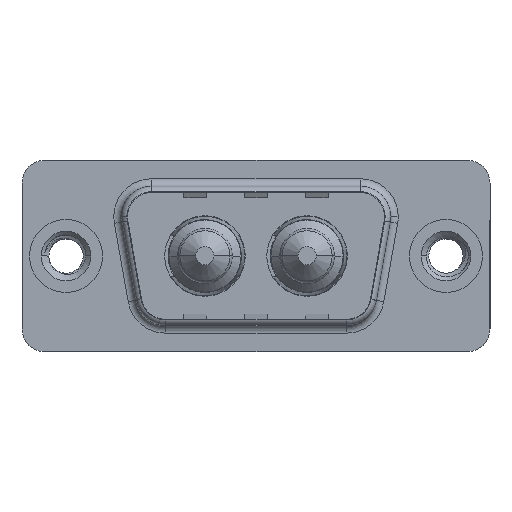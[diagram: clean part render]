
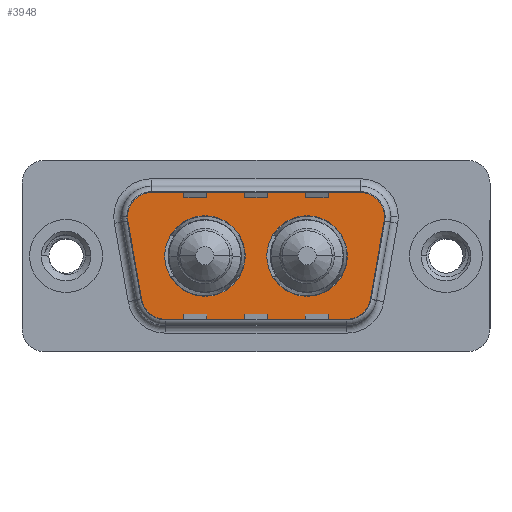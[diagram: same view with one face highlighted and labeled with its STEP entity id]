
A CAD part, top view. The second image highlights one B-rep face of the part: STEP entity #3948.
In plain terms, the highlighted planar face has unit normal (0, 0, 1).
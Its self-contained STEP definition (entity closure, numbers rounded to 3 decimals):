
#132 = CARTESIAN_POINT ( 'NONE',  ( 5.436, 2.9, 0. ) ) ;
#483 = FACE_OUTER_BOUND ( 'NONE', #4924, .T. ) ;
#652 = CARTESIAN_POINT ( 'NONE',  ( 18.51, 0., 0. ) ) ;
#672 = DIRECTION ( 'NONE',  ( 0., 0., 1. ) ) ;
#701 = DIRECTION ( 'NONE',  ( 1., 0., 0. ) ) ;
#782 = VERTEX_POINT ( 'NONE', #12612 ) ;
#841 = EDGE_CURVE ( 'NONE', #10026, #9860, #6600, .T. ) ;
#911 = CARTESIAN_POINT ( 'NONE',  ( 9.14, 0., 0. ) ) ;
#1063 = DIRECTION ( 'NONE',  ( 0., 0., 1. ) ) ;
#1115 = EDGE_CURVE ( 'NONE', #13085, #6826, #3585, .T. ) ;
#1200 = AXIS2_PLACEMENT_3D ( 'NONE', #3878, #1221, #13294 ) ;
#1221 = DIRECTION ( 'NONE',  ( 0., 0., 1. ) ) ;
#1345 = DIRECTION ( 'NONE',  ( 1., 0., 0. ) ) ;
#1602 = ORIENTED_EDGE ( 'NONE', *, *, #3446, .T. ) ;
#1955 = DIRECTION ( 'NONE',  ( 0., 0., 1. ) ) ;
#2204 = CARTESIAN_POINT ( 'NONE',  ( 3.466, 2.553, 0. ) ) ;
#2208 = CARTESIAN_POINT ( 'NONE',  ( 20.511, -3.247, 0. ) ) ;
#2267 = DIRECTION ( 'NONE',  ( -1., 0., 0. ) ) ;
#2275 = PLANE ( 'NONE',  #1200 ) ;
#2322 = ORIENTED_EDGE ( 'NONE', *, *, #5563, .F. ) ;
#2323 = VERTEX_POINT ( 'NONE', #7540 ) ;
#2483 = CARTESIAN_POINT ( 'NONE',  ( 19.564, 2.9, 0. ) ) ;
#2582 = LINE ( 'NONE', #13268, #15132 ) ;
#2843 = CARTESIAN_POINT ( 'NONE',  ( 4.489, -3.247, 0. ) ) ;
#2869 = EDGE_CURVE ( 'NONE', #10676, #13154, #8238, .T. ) ;
#2882 = CIRCLE ( 'NONE', #6363, 2. ) ;
#2895 = CIRCLE ( 'NONE', #12965, 2.65 ) ;
#3183 = CIRCLE ( 'NONE', #9169, 2. ) ;
#3239 = ORIENTED_EDGE ( 'NONE', *, *, #841, .T. ) ;
#3446 = EDGE_CURVE ( 'NONE', #6826, #2323, #2582, .T. ) ;
#3585 = CIRCLE ( 'NONE', #12655, 2. ) ;
#3688 = ORIENTED_EDGE ( 'NONE', *, *, #4561, .T. ) ;
#3711 = FACE_BOUND ( 'NONE', #8739, .T. ) ;
#3712 = DIRECTION ( 'NONE',  ( -1., 0., 0. ) ) ;
#3720 = CARTESIAN_POINT ( 'NONE',  ( 15.86, 0., 0. ) ) ;
#3811 = DIRECTION ( 'NONE',  ( 0., 0., 1. ) ) ;
#3878 = CARTESIAN_POINT ( 'NONE',  ( 18.541, -2.9, 0. ) ) ;
#3948 = ADVANCED_FACE ( 'NONE', ( #13364, #3711, #483 ), #2275, .T. ) ;
#4090 = CARTESIAN_POINT ( 'NONE',  ( 5.436, 4.9, 0. ) ) ;
#4270 = CARTESIAN_POINT ( 'NONE',  ( 11.79, 0., 0. ) ) ;
#4561 = EDGE_CURVE ( 'NONE', #782, #10026, #7264, .T. ) ;
#4793 = CARTESIAN_POINT ( 'NONE',  ( 6.49, 0., 0. ) ) ;
#4800 = CIRCLE ( 'NONE', #15759, 2. ) ;
#4924 = EDGE_LOOP ( 'NONE', ( #15242, #1602, #11312, #3688, #3239, #15595, #5455, #5734, #7598 ) ) ;
#4936 = DIRECTION ( 'NONE',  ( 1., 0., 0. ) ) ;
#5147 = AXIS2_PLACEMENT_3D ( 'NONE', #8876, #11885, #11866 ) ;
#5151 = VERTEX_POINT ( 'NONE', #4793 ) ;
#5455 = ORIENTED_EDGE ( 'NONE', *, *, #2869, .T. ) ;
#5510 = DIRECTION ( 'NONE',  ( 0.174, -0.985, 0. ) ) ;
#5563 = EDGE_CURVE ( 'NONE', #8198, #10175, #7054, .T. ) ;
#5567 = VERTEX_POINT ( 'NONE', #4270 ) ;
#5734 = ORIENTED_EDGE ( 'NONE', *, *, #6696, .T. ) ;
#5757 = EDGE_CURVE ( 'NONE', #2323, #782, #4800, .T. ) ;
#5960 = DIRECTION ( 'NONE',  ( 1., 0., 0. ) ) ;
#5963 = EDGE_CURVE ( 'NONE', #5151, #5567, #2895, .T. ) ;
#6213 = VECTOR ( 'NONE', #2267, 1000. ) ;
#6236 = CARTESIAN_POINT ( 'NONE',  ( 3.466, 2.553, 0. ) ) ;
#6363 = AXIS2_PLACEMENT_3D ( 'NONE', #6787, #6740, #6719 ) ;
#6600 = LINE ( 'NONE', #15587, #6213 ) ;
#6684 = VERTEX_POINT ( 'NONE', #7720 ) ;
#6696 = EDGE_CURVE ( 'NONE', #13154, #6684, #2882, .T. ) ;
#6719 = DIRECTION ( 'NONE',  ( -1., 0., 0. ) ) ;
#6740 = DIRECTION ( 'NONE',  ( 0., 0., 1. ) ) ;
#6787 = CARTESIAN_POINT ( 'NONE',  ( 6.459, -2.9, 0. ) ) ;
#6826 = VERTEX_POINT ( 'NONE', #2208 ) ;
#7026 = CARTESIAN_POINT ( 'NONE',  ( 6.459, -4.9, 0. ) ) ;
#7054 = CIRCLE ( 'NONE', #5147, 2.65 ) ;
#7264 = CIRCLE ( 'NONE', #12854, 2. ) ;
#7540 = CARTESIAN_POINT ( 'NONE',  ( 21.534, 2.553, 0. ) ) ;
#7598 = ORIENTED_EDGE ( 'NONE', *, *, #8894, .T. ) ;
#7692 = VECTOR ( 'NONE', #5960, 1000. ) ;
#7720 = CARTESIAN_POINT ( 'NONE',  ( 6.459, -4.9, 0. ) ) ;
#7918 = EDGE_CURVE ( 'NONE', #9860, #10676, #3183, .T. ) ;
#8198 = VERTEX_POINT ( 'NONE', #652 ) ;
#8238 = LINE ( 'NONE', #6236, #14755 ) ;
#8577 = DIRECTION ( 'NONE',  ( 0., 0., 1. ) ) ;
#8739 = EDGE_LOOP ( 'NONE', ( #12977, #15034 ) ) ;
#8876 = CARTESIAN_POINT ( 'NONE',  ( 15.86, 0., 0. ) ) ;
#8894 = EDGE_CURVE ( 'NONE', #6684, #13085, #15540, .T. ) ;
#9168 = CARTESIAN_POINT ( 'NONE',  ( 9.14, 0., 0. ) ) ;
#9169 = AXIS2_PLACEMENT_3D ( 'NONE', #132, #8577, #1345 ) ;
#9634 = EDGE_LOOP ( 'NONE', ( #2322, #14227 ) ) ;
#9860 = VERTEX_POINT ( 'NONE', #4090 ) ;
#9920 = EDGE_CURVE ( 'NONE', #5567, #5151, #12270, .T. ) ;
#10026 = VERTEX_POINT ( 'NONE', #14216 ) ;
#10175 = VERTEX_POINT ( 'NONE', #10807 ) ;
#10211 = EDGE_CURVE ( 'NONE', #10175, #8198, #12448, .T. ) ;
#10396 = DIRECTION ( 'NONE',  ( 1., 0., 0. ) ) ;
#10676 = VERTEX_POINT ( 'NONE', #2204 ) ;
#10807 = CARTESIAN_POINT ( 'NONE',  ( 13.21, 0., 0. ) ) ;
#11076 = DIRECTION ( 'NONE',  ( 0.174, 0.985, 0. ) ) ;
#11312 = ORIENTED_EDGE ( 'NONE', *, *, #5757, .T. ) ;
#11548 = DIRECTION ( 'NONE',  ( 1., 0., 0. ) ) ;
#11866 = DIRECTION ( 'NONE',  ( 1., 0., 0. ) ) ;
#11885 = DIRECTION ( 'NONE',  ( 0., 0., 1. ) ) ;
#12060 = CARTESIAN_POINT ( 'NONE',  ( 18.541, -2.9, 0. ) ) ;
#12096 = DIRECTION ( 'NONE',  ( 0., 0., 1. ) ) ;
#12191 = DIRECTION ( 'NONE',  ( 0., 0., 1. ) ) ;
#12270 = CIRCLE ( 'NONE', #13014, 2.65 ) ;
#12280 = CARTESIAN_POINT ( 'NONE',  ( 18.541, -4.9, 0. ) ) ;
#12448 = CIRCLE ( 'NONE', #15240, 2.65 ) ;
#12612 = CARTESIAN_POINT ( 'NONE',  ( 21.564, 2.9, 0. ) ) ;
#12655 = AXIS2_PLACEMENT_3D ( 'NONE', #12060, #12096, #11548 ) ;
#12854 = AXIS2_PLACEMENT_3D ( 'NONE', #2483, #3811, #3712 ) ;
#12965 = AXIS2_PLACEMENT_3D ( 'NONE', #911, #1063, #701 ) ;
#12977 = ORIENTED_EDGE ( 'NONE', *, *, #9920, .F. ) ;
#13014 = AXIS2_PLACEMENT_3D ( 'NONE', #9168, #1955, #10396 ) ;
#13085 = VERTEX_POINT ( 'NONE', #12280 ) ;
#13154 = VERTEX_POINT ( 'NONE', #2843 ) ;
#13268 = CARTESIAN_POINT ( 'NONE',  ( 21.534, 2.553, 0. ) ) ;
#13294 = DIRECTION ( 'NONE',  ( 1., 0., 0. ) ) ;
#13364 = FACE_BOUND ( 'NONE', #9634, .T. ) ;
#13687 = DIRECTION ( 'NONE',  ( -1., 0., 0. ) ) ;
#14216 = CARTESIAN_POINT ( 'NONE',  ( 19.564, 4.9, 0. ) ) ;
#14227 = ORIENTED_EDGE ( 'NONE', *, *, #10211, .F. ) ;
#14294 = CARTESIAN_POINT ( 'NONE',  ( 19.564, 2.9, 0. ) ) ;
#14755 = VECTOR ( 'NONE', #5510, 1000. ) ;
#15034 = ORIENTED_EDGE ( 'NONE', *, *, #5963, .F. ) ;
#15132 = VECTOR ( 'NONE', #11076, 1000. ) ;
#15240 = AXIS2_PLACEMENT_3D ( 'NONE', #3720, #12191, #4936 ) ;
#15242 = ORIENTED_EDGE ( 'NONE', *, *, #1115, .T. ) ;
#15540 = LINE ( 'NONE', #7026, #7692 ) ;
#15587 = CARTESIAN_POINT ( 'NONE',  ( 5.436, 4.9, 0. ) ) ;
#15595 = ORIENTED_EDGE ( 'NONE', *, *, #7918, .T. ) ;
#15759 = AXIS2_PLACEMENT_3D ( 'NONE', #14294, #672, #13687 ) ;
